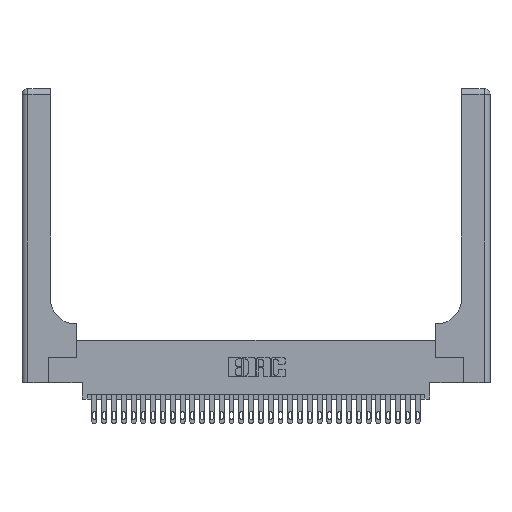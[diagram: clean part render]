
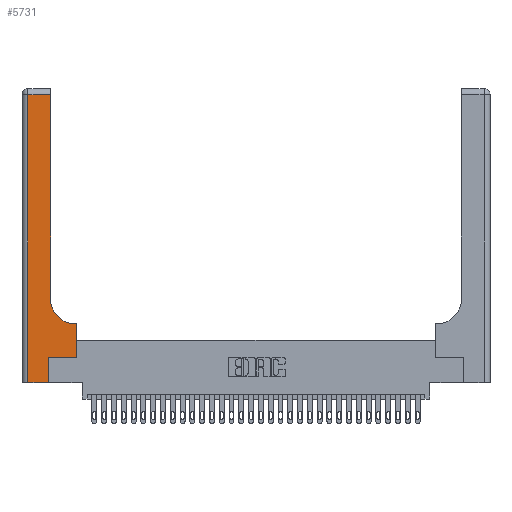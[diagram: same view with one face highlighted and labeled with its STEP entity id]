
A CAD part, top view. The second image highlights one B-rep face of the part: STEP entity #5731.
In plain terms, the highlighted planar face has unit normal (0, 0, 1).
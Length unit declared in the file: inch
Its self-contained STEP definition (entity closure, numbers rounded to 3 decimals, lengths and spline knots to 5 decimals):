
#251 = EDGE_CURVE ( 'NONE', #27345, #16066, #25085, .T. ) ;
#800 = CARTESIAN_POINT ( 'NONE',  ( 0.06, 3., 0.37 ) ) ;
#1122 = VECTOR ( 'NONE', #2575, 39.37008 ) ;
#1330 = CARTESIAN_POINT ( 'NONE',  ( 0.269, 0., 0.37 ) ) ;
#1592 = CARTESIAN_POINT ( 'NONE',  ( 0.269, 0.25, 0.37 ) ) ;
#2241 = AXIS2_PLACEMENT_3D ( 'NONE', #30104, #12356, #3015 ) ;
#2547 = VERTEX_POINT ( 'NONE', #22025 ) ;
#2575 = DIRECTION ( 'NONE',  ( 0., 1., 0. ) ) ;
#2965 = VECTOR ( 'NONE', #19522, 39.37008 ) ;
#3015 = DIRECTION ( 'NONE',  ( -1., 0., 0. ) ) ;
#3267 = EDGE_CURVE ( 'NONE', #2547, #7277, #26103, .T. ) ;
#3353 = EDGE_CURVE ( 'NONE', #7359, #24937, #12896, .T. ) ;
#4876 = LINE ( 'NONE', #800, #24462 ) ;
#5656 = EDGE_CURVE ( 'NONE', #20815, #7359, #4876, .T. ) ;
#5731 = ADVANCED_FACE ( 'NONE', ( #10406 ), #12134, .F. ) ;
#5853 = EDGE_CURVE ( 'NONE', #24937, #2547, #27225, .T. ) ;
#6807 = CARTESIAN_POINT ( 'NONE',  ( 0.2915, 2.94, 0.37 ) ) ;
#7277 = VERTEX_POINT ( 'NONE', #12776 ) ;
#7359 = VERTEX_POINT ( 'NONE', #21507 ) ;
#7868 = VECTOR ( 'NONE', #18100, 39.37008 ) ;
#9549 = VECTOR ( 'NONE', #27065, 39.37008 ) ;
#9959 = DIRECTION ( 'NONE',  ( 1., 0., 0. ) ) ;
#10315 = CARTESIAN_POINT ( 'NONE',  ( 0.2915, 3., 0.37 ) ) ;
#10406 = FACE_OUTER_BOUND ( 'NONE', #25577, .T. ) ;
#10834 = ORIENTED_EDGE ( 'NONE', *, *, #31310, .T. ) ;
#11933 = ORIENTED_EDGE ( 'NONE', *, *, #19767, .T. ) ;
#12033 = EDGE_CURVE ( 'NONE', #7277, #14713, #14735, .T. ) ;
#12134 = PLANE ( 'NONE',  #2241 ) ;
#12347 = DIRECTION ( 'NONE',  ( -1., 0., 0. ) ) ;
#12356 = DIRECTION ( 'NONE',  ( 0., 0., -1. ) ) ;
#12453 = CARTESIAN_POINT ( 'NONE',  ( 0.2915, 0.85, 0.37 ) ) ;
#12776 = CARTESIAN_POINT ( 'NONE',  ( 0.5585, 0.25, 0.37 ) ) ;
#12896 = LINE ( 'NONE', #20266, #25687 ) ;
#12982 = CARTESIAN_POINT ( 'NONE',  ( 0., 2.94, 0.37 ) ) ;
#13424 = ORIENTED_EDGE ( 'NONE', *, *, #3267, .T. ) ;
#13435 = ORIENTED_EDGE ( 'NONE', *, *, #5656, .T. ) ;
#14239 = DIRECTION ( 'NONE',  ( 0., 1., 0. ) ) ;
#14618 = LINE ( 'NONE', #27657, #28580 ) ;
#14655 = DIRECTION ( 'NONE',  ( 1., 0., 0. ) ) ;
#14713 = VERTEX_POINT ( 'NONE', #24593 ) ;
#14735 = LINE ( 'NONE', #29717, #9549 ) ;
#15455 = LINE ( 'NONE', #12982, #7868 ) ;
#16066 = VERTEX_POINT ( 'NONE', #6807 ) ;
#17021 = CARTESIAN_POINT ( 'NONE',  ( 0.5415, 0.85, 0.37 ) ) ;
#18100 = DIRECTION ( 'NONE',  ( -1., 0., 0. ) ) ;
#19522 = DIRECTION ( 'NONE',  ( 1., 0., 0. ) ) ;
#19699 = DIRECTION ( 'NONE',  ( 0., 0., -1. ) ) ;
#19767 = EDGE_CURVE ( 'NONE', #16066, #20815, #15455, .T. ) ;
#20266 = CARTESIAN_POINT ( 'NONE',  ( 0., 0., 0.37 ) ) ;
#20815 = VERTEX_POINT ( 'NONE', #27880 ) ;
#21466 = ORIENTED_EDGE ( 'NONE', *, *, #251, .T. ) ;
#21507 = CARTESIAN_POINT ( 'NONE',  ( 0.06, 0., 0.37 ) ) ;
#22025 = CARTESIAN_POINT ( 'NONE',  ( 0.269, 0.25, 0.37 ) ) ;
#22046 = VECTOR ( 'NONE', #14239, 39.37008 ) ;
#23190 = ORIENTED_EDGE ( 'NONE', *, *, #12033, .T. ) ;
#24278 = AXIS2_PLACEMENT_3D ( 'NONE', #17021, #19699, #14655 ) ;
#24462 = VECTOR ( 'NONE', #29467, 39.37008 ) ;
#24593 = CARTESIAN_POINT ( 'NONE',  ( 0.5585, 0.6, 0.37 ) ) ;
#24937 = VERTEX_POINT ( 'NONE', #25797 ) ;
#25085 = LINE ( 'NONE', #10315, #1122 ) ;
#25175 = ORIENTED_EDGE ( 'NONE', *, *, #5853, .T. ) ;
#25321 = ORIENTED_EDGE ( 'NONE', *, *, #28898, .T. ) ;
#25577 = EDGE_LOOP ( 'NONE', ( #21466, #11933, #13435, #31509, #25175, #13424, #23190, #25321, #10834 ) ) ;
#25687 = VECTOR ( 'NONE', #9959, 39.37008 ) ;
#25797 = CARTESIAN_POINT ( 'NONE',  ( 0.269, 0., 0.37 ) ) ;
#26103 = LINE ( 'NONE', #1592, #2965 ) ;
#27065 = DIRECTION ( 'NONE',  ( 0., 1., 0. ) ) ;
#27225 = LINE ( 'NONE', #1330, #22046 ) ;
#27345 = VERTEX_POINT ( 'NONE', #12453 ) ;
#27657 = CARTESIAN_POINT ( 'NONE',  ( 0.2915, 0.6, 0.37 ) ) ;
#27880 = CARTESIAN_POINT ( 'NONE',  ( 0.06, 2.94, 0.37 ) ) ;
#28130 = VERTEX_POINT ( 'NONE', #31262 ) ;
#28580 = VECTOR ( 'NONE', #12347, 39.37008 ) ;
#28898 = EDGE_CURVE ( 'NONE', #14713, #28130, #14618, .T. ) ;
#29467 = DIRECTION ( 'NONE',  ( 0., -1., 0. ) ) ;
#29717 = CARTESIAN_POINT ( 'NONE',  ( 0.5585, 0.25, 0.37 ) ) ;
#30104 = CARTESIAN_POINT ( 'NONE',  ( 0., 3., 0.37 ) ) ;
#31262 = CARTESIAN_POINT ( 'NONE',  ( 0.5415, 0.6, 0.37 ) ) ;
#31310 = EDGE_CURVE ( 'NONE', #28130, #27345, #32724, .T. ) ;
#31509 = ORIENTED_EDGE ( 'NONE', *, *, #3353, .T. ) ;
#32724 = CIRCLE ( 'NONE', #24278, 0.25 ) ;
